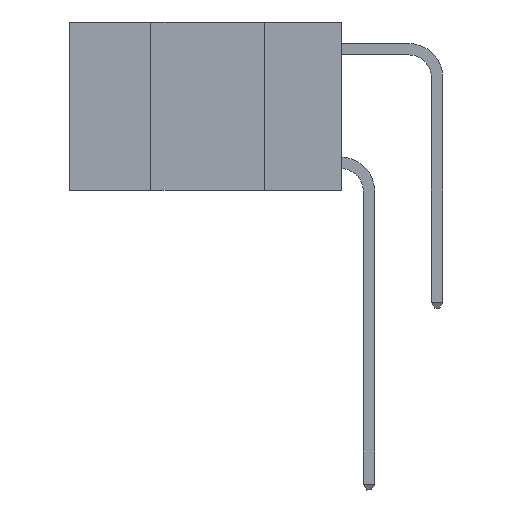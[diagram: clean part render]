
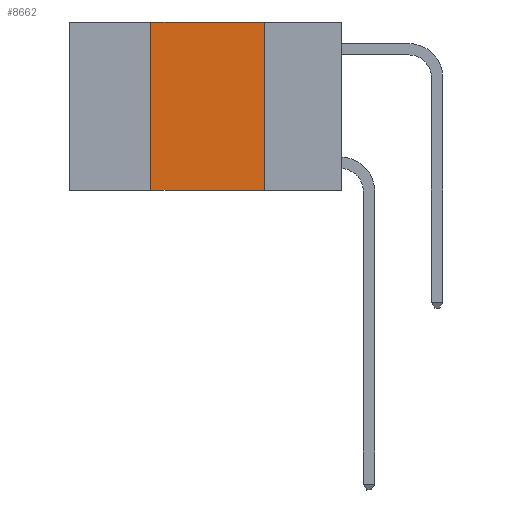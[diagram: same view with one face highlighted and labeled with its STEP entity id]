
A CAD part, left-side view. The second image highlights one B-rep face of the part: STEP entity #8662.
In plain terms, the highlighted planar face has unit normal (-1, 0, 0).
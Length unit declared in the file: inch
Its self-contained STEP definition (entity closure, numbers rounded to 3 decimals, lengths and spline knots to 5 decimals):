
#434 = DIRECTION ( 'NONE',  ( 1., 0., 0. ) ) ;
#1369 = DIRECTION ( 'NONE',  ( 0., -1., 0. ) ) ;
#1971 = CARTESIAN_POINT ( 'NONE',  ( 0., 0.42, -0.37 ) ) ;
#2284 = VECTOR ( 'NONE', #1369, 39.37008 ) ;
#2634 = LINE ( 'NONE', #5743, #4879 ) ;
#3539 = CARTESIAN_POINT ( 'NONE',  ( 0., 0.17, 0. ) ) ;
#3665 = EDGE_CURVE ( 'NONE', #3777, #7444, #13218, .T. ) ;
#3684 = EDGE_CURVE ( 'NONE', #9028, #7444, #7884, .T. ) ;
#3687 = EDGE_CURVE ( 'NONE', #9028, #8800, #2634, .T. ) ;
#3777 = VERTEX_POINT ( 'NONE', #5912 ) ;
#3879 = CARTESIAN_POINT ( 'NONE',  ( 0., 0.17, -0.37 ) ) ;
#4761 = EDGE_CURVE ( 'NONE', #8800, #3777, #10156, .T. ) ;
#4850 = VECTOR ( 'NONE', #10847, 39.37008 ) ;
#4879 = VECTOR ( 'NONE', #9697, 39.37008 ) ;
#5743 = CARTESIAN_POINT ( 'NONE',  ( 0., 0.42, 0. ) ) ;
#5839 = FACE_OUTER_BOUND ( 'NONE', #9105, .T. ) ;
#5898 = ORIENTED_EDGE ( 'NONE', *, *, #3665, .F. ) ;
#5912 = CARTESIAN_POINT ( 'NONE',  ( 0., 0.17, 0. ) ) ;
#6001 = ORIENTED_EDGE ( 'NONE', *, *, #4761, .F. ) ;
#6081 = ORIENTED_EDGE ( 'NONE', *, *, #3687, .F. ) ;
#6094 = CARTESIAN_POINT ( 'NONE',  ( 0., 0.42, 0. ) ) ;
#6324 = ORIENTED_EDGE ( 'NONE', *, *, #3684, .T. ) ;
#6904 = CARTESIAN_POINT ( 'NONE',  ( 0., 0.6, 0. ) ) ;
#6940 = CARTESIAN_POINT ( 'NONE',  ( 0., 0.6, 0. ) ) ;
#7444 = VERTEX_POINT ( 'NONE', #3879 ) ;
#7773 = CARTESIAN_POINT ( 'NONE',  ( 0., 0.6, -0.37 ) ) ;
#7884 = LINE ( 'NONE', #7773, #2284 ) ;
#7996 = DIRECTION ( 'NONE',  ( 0., 0., -1. ) ) ;
#8662 = ADVANCED_FACE ( 'NONE', ( #5839 ), #10880, .F. ) ;
#8682 = DIRECTION ( 'NONE',  ( 0., 0., -1. ) ) ;
#8800 = VERTEX_POINT ( 'NONE', #6094 ) ;
#9028 = VERTEX_POINT ( 'NONE', #1971 ) ;
#9105 = EDGE_LOOP ( 'NONE', ( #5898, #6001, #6081, #6324 ) ) ;
#9697 = DIRECTION ( 'NONE',  ( 0., 0., 1. ) ) ;
#10156 = LINE ( 'NONE', #6904, #4850 ) ;
#10847 = DIRECTION ( 'NONE',  ( 0., -1., 0. ) ) ;
#10880 = PLANE ( 'NONE',  #11745 ) ;
#11745 = AXIS2_PLACEMENT_3D ( 'NONE', #6940, #434, #7996 ) ;
#12931 = VECTOR ( 'NONE', #8682, 39.37008 ) ;
#13218 = LINE ( 'NONE', #3539, #12931 ) ;
